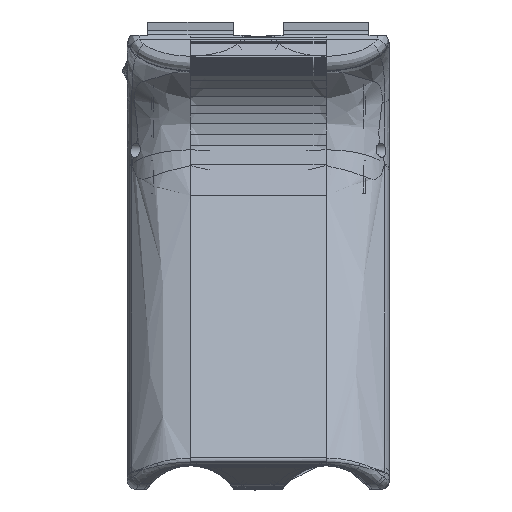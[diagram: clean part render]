
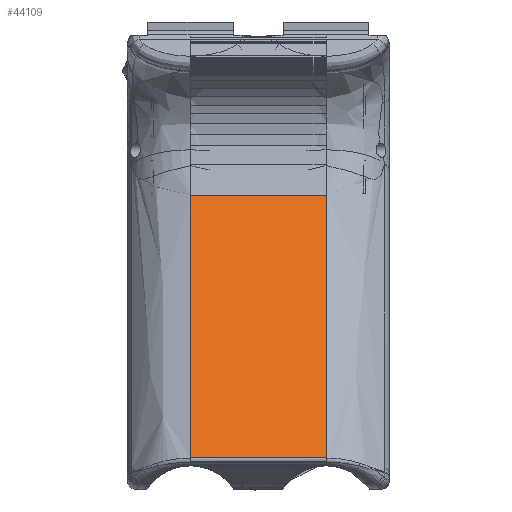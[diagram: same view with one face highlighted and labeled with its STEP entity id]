
A CAD part, left-side view. The second image highlights one B-rep face of the part: STEP entity #44109.
In plain terms, the highlighted planar face has unit normal (-0.93, 0, 0.366).
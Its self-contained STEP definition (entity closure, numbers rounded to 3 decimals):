
#6568=FACE_OUTER_BOUND('',#9000,.T.);
#9000=EDGE_LOOP('',(#39407,#39408,#39409,#39410));
#11898=LINE('',#138364,#15488);
#12210=LINE('',#140842,#15800);
#12211=LINE('',#140845,#15801);
#12212=LINE('',#140846,#15802);
#15488=VECTOR('',#54557,10.);
#15800=VECTOR('',#55051,10.);
#15801=VECTOR('',#55054,10.);
#15802=VECTOR('',#55055,10.);
#19980=VERTEX_POINT('',#138349);
#19981=VERTEX_POINT('',#138363);
#20270=VERTEX_POINT('',#140828);
#20271=VERTEX_POINT('',#140844);
#26304=EDGE_CURVE('',#19981,#19980,#11898,.T.);
#26743=EDGE_CURVE('',#19980,#20270,#12210,.T.);
#26744=EDGE_CURVE('',#20271,#20270,#12211,.T.);
#26745=EDGE_CURVE('',#19981,#20271,#12212,.T.);
#39407=ORIENTED_EDGE('',*,*,#26304,.T.);
#39408=ORIENTED_EDGE('',*,*,#26743,.T.);
#39409=ORIENTED_EDGE('',*,*,#26744,.F.);
#39410=ORIENTED_EDGE('',*,*,#26745,.F.);
#41744=PLANE('',#46844);
#44109=ADVANCED_FACE('',(#6568),#41744,.T.);
#46844=AXIS2_PLACEMENT_3D('',#140843,#55052,#55053);
#54557=DIRECTION('',(-0.367,0.,-0.93));
#55051=DIRECTION('',(0.,-1.,0.));
#55052=DIRECTION('center_axis',(-0.93,0.,
0.367));
#55053=DIRECTION('ref_axis',(-0.367,0.,-0.93));
#55054=DIRECTION('',(-0.367,0.,-0.93));
#55055=DIRECTION('',(0.,-1.,0.));
#138349=CARTESIAN_POINT('',(-89.309,56.48,7.104));
#138363=CARTESIAN_POINT('',(-65.769,56.48,66.865));
#138364=CARTESIAN_POINT('',(-61.718,56.48,77.148));
#140828=CARTESIAN_POINT('',(-89.309,25.48,7.104));
#140842=CARTESIAN_POINT('',(-89.309,56.48,7.104));
#140843=CARTESIAN_POINT('Origin',(-65.769,56.48,66.865));
#140844=CARTESIAN_POINT('',(-65.769,25.48,66.865));
#140845=CARTESIAN_POINT('',(-61.718,25.48,77.148));
#140846=CARTESIAN_POINT('',(-65.769,56.48,66.865));
